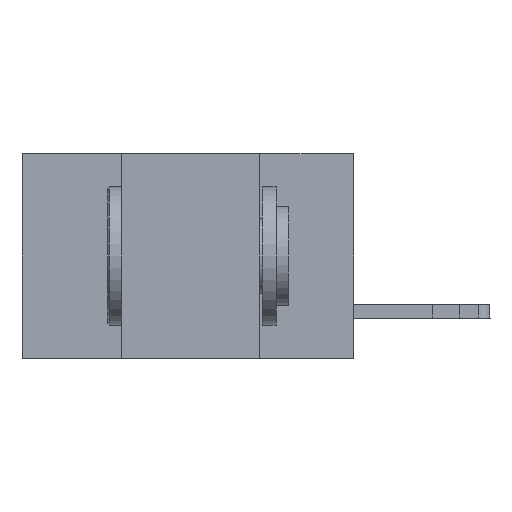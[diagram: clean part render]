
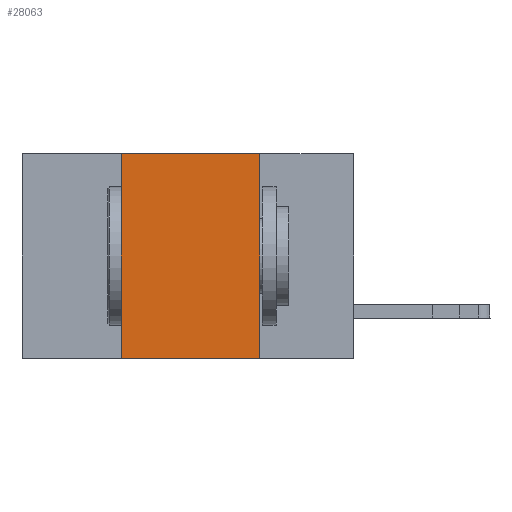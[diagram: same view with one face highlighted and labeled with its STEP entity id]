
A CAD part, left-side view. The second image highlights one B-rep face of the part: STEP entity #28063.
In plain terms, the highlighted planar face has unit normal (-1, 0, 0).
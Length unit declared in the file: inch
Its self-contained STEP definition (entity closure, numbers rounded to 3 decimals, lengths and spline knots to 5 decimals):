
#529 = CARTESIAN_POINT ( 'NONE',  ( 0., 0.42, 0. ) ) ;
#1574 = EDGE_CURVE ( 'NONE', #10902, #6460, #18416, .T. ) ;
#1640 = VECTOR ( 'NONE', #34939, 39.37008 ) ;
#2897 = VECTOR ( 'NONE', #23432, 39.37008 ) ;
#4763 = DIRECTION ( 'NONE',  ( 1., 0., 0. ) ) ;
#5864 = LINE ( 'NONE', #14525, #7203 ) ;
#6337 = PLANE ( 'NONE',  #30258 ) ;
#6460 = VERTEX_POINT ( 'NONE', #11479 ) ;
#7203 = VECTOR ( 'NONE', #17330, 39.37008 ) ;
#7909 = DIRECTION ( 'NONE',  ( 0., 0., -1. ) ) ;
#8145 = LINE ( 'NONE', #529, #2897 ) ;
#10494 = ORIENTED_EDGE ( 'NONE', *, *, #14131, .F. ) ;
#10902 = VERTEX_POINT ( 'NONE', #19951 ) ;
#11479 = CARTESIAN_POINT ( 'NONE',  ( 0., 0.17, -0.37 ) ) ;
#11886 = VERTEX_POINT ( 'NONE', #31424 ) ;
#12724 = DIRECTION ( 'NONE',  ( 0., -1., 0. ) ) ;
#14131 = EDGE_CURVE ( 'NONE', #11886, #34093, #26908, .T. ) ;
#14525 = CARTESIAN_POINT ( 'NONE',  ( 0., 0.17, 0. ) ) ;
#16562 = CARTESIAN_POINT ( 'NONE',  ( 0., 0.17, 0. ) ) ;
#17330 = DIRECTION ( 'NONE',  ( 0., 0., -1. ) ) ;
#17923 = CARTESIAN_POINT ( 'NONE',  ( 0., 0.6, 0. ) ) ;
#18416 = LINE ( 'NONE', #23845, #19682 ) ;
#18533 = CARTESIAN_POINT ( 'NONE',  ( 0., 0.6, 0. ) ) ;
#18867 = ORIENTED_EDGE ( 'NONE', *, *, #27355, .F. ) ;
#19447 = ORIENTED_EDGE ( 'NONE', *, *, #26350, .F. ) ;
#19682 = VECTOR ( 'NONE', #12724, 39.37008 ) ;
#19951 = CARTESIAN_POINT ( 'NONE',  ( 0., 0.42, -0.37 ) ) ;
#20254 = ORIENTED_EDGE ( 'NONE', *, *, #1574, .T. ) ;
#21060 = FACE_OUTER_BOUND ( 'NONE', #33866, .T. ) ;
#23432 = DIRECTION ( 'NONE',  ( 0., 0., 1. ) ) ;
#23845 = CARTESIAN_POINT ( 'NONE',  ( 0., 0.6, -0.37 ) ) ;
#26350 = EDGE_CURVE ( 'NONE', #10902, #11886, #8145, .T. ) ;
#26908 = LINE ( 'NONE', #17923, #1640 ) ;
#27355 = EDGE_CURVE ( 'NONE', #34093, #6460, #5864, .T. ) ;
#28063 = ADVANCED_FACE ( 'NONE', ( #21060 ), #6337, .F. ) ;
#30258 = AXIS2_PLACEMENT_3D ( 'NONE', #18533, #4763, #7909 ) ;
#31424 = CARTESIAN_POINT ( 'NONE',  ( 0., 0.42, 0. ) ) ;
#33866 = EDGE_LOOP ( 'NONE', ( #18867, #10494, #19447, #20254 ) ) ;
#34093 = VERTEX_POINT ( 'NONE', #16562 ) ;
#34939 = DIRECTION ( 'NONE',  ( 0., -1., 0. ) ) ;
